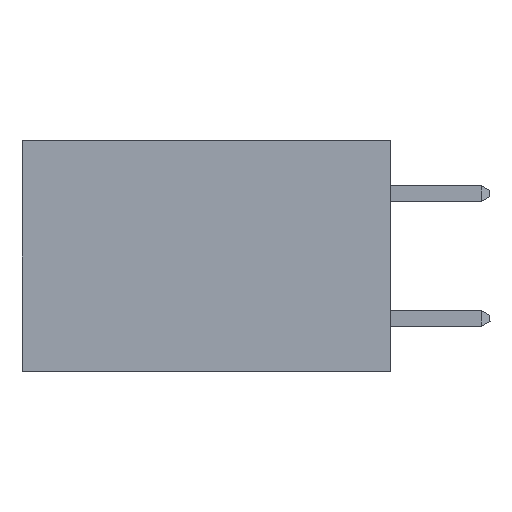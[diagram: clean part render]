
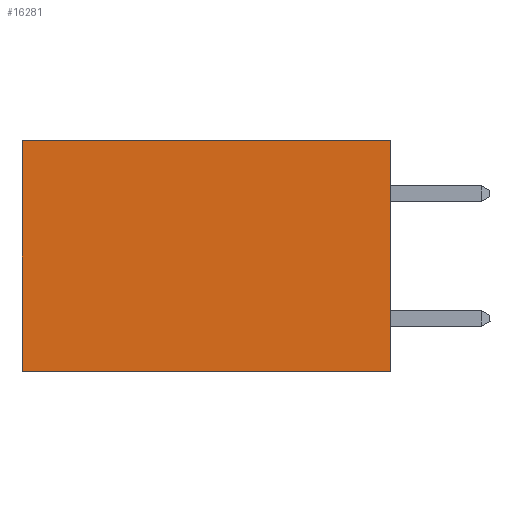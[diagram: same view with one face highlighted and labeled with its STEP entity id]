
A CAD part, left-side view. The second image highlights one B-rep face of the part: STEP entity #16281.
In plain terms, the highlighted planar face has unit normal (-1, 0, 0).
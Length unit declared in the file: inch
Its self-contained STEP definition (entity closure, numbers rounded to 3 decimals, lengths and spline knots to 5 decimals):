
#128 = DIRECTION ( 'NONE',  ( 0., 0., -1. ) ) ;
#257 = CARTESIAN_POINT ( 'NONE',  ( 0.277, 0., -0.37 ) ) ;
#2141 = EDGE_CURVE ( 'NONE', #23148, #18848, #10583, .T. ) ;
#3123 = CARTESIAN_POINT ( 'NONE',  ( 0.277, 0.59, 0. ) ) ;
#4515 = VECTOR ( 'NONE', #25559, 39.37008 ) ;
#4803 = CARTESIAN_POINT ( 'NONE',  ( 0.277, 0., -0.37 ) ) ;
#5555 = VERTEX_POINT ( 'NONE', #10475 ) ;
#5620 = ORIENTED_EDGE ( 'NONE', *, *, #5766, .F. ) ;
#5766 = EDGE_CURVE ( 'NONE', #23148, #12431, #15302, .T. ) ;
#6396 = DIRECTION ( 'NONE',  ( 0., 0., -1. ) ) ;
#6499 = CARTESIAN_POINT ( 'NONE',  ( 0.277, 0., -0.37 ) ) ;
#6971 = CARTESIAN_POINT ( 'NONE',  ( 0.277, 0., -0.37 ) ) ;
#7122 = DIRECTION ( 'NONE',  ( 1., 0., 0. ) ) ;
#7481 = VECTOR ( 'NONE', #6396, 39.37008 ) ;
#7839 = VECTOR ( 'NONE', #128, 39.37008 ) ;
#9259 = DIRECTION ( 'NONE',  ( 0., 1., 0. ) ) ;
#10475 = CARTESIAN_POINT ( 'NONE',  ( 0.277, 0.59, -0.37 ) ) ;
#10566 = ORIENTED_EDGE ( 'NONE', *, *, #24599, .F. ) ;
#10583 = LINE ( 'NONE', #24384, #4515 ) ;
#11208 = LINE ( 'NONE', #6971, #22483 ) ;
#12431 = VERTEX_POINT ( 'NONE', #6499 ) ;
#12695 = ORIENTED_EDGE ( 'NONE', *, *, #2141, .T. ) ;
#13527 = LINE ( 'NONE', #28979, #7481 ) ;
#15302 = LINE ( 'NONE', #257, #7839 ) ;
#15303 = EDGE_LOOP ( 'NONE', ( #15680, #10566, #5620, #12695 ) ) ;
#15680 = ORIENTED_EDGE ( 'NONE', *, *, #18478, .T. ) ;
#16281 = ADVANCED_FACE ( 'NONE', ( #17831 ), #20667, .F. ) ;
#17831 = FACE_OUTER_BOUND ( 'NONE', #15303, .T. ) ;
#18478 = EDGE_CURVE ( 'NONE', #18848, #5555, #13527, .T. ) ;
#18848 = VERTEX_POINT ( 'NONE', #3123 ) ;
#20667 = PLANE ( 'NONE',  #29135 ) ;
#22483 = VECTOR ( 'NONE', #9259, 39.37008 ) ;
#22932 = DIRECTION ( 'NONE',  ( 0., 0., -1. ) ) ;
#23148 = VERTEX_POINT ( 'NONE', #27060 ) ;
#24384 = CARTESIAN_POINT ( 'NONE',  ( 0.277, 0., 0. ) ) ;
#24599 = EDGE_CURVE ( 'NONE', #12431, #5555, #11208, .T. ) ;
#25559 = DIRECTION ( 'NONE',  ( 0., 1., 0. ) ) ;
#27060 = CARTESIAN_POINT ( 'NONE',  ( 0.277, 0., 0. ) ) ;
#28979 = CARTESIAN_POINT ( 'NONE',  ( 0.277, 0.59, -0.37 ) ) ;
#29135 = AXIS2_PLACEMENT_3D ( 'NONE', #4803, #7122, #22932 ) ;
